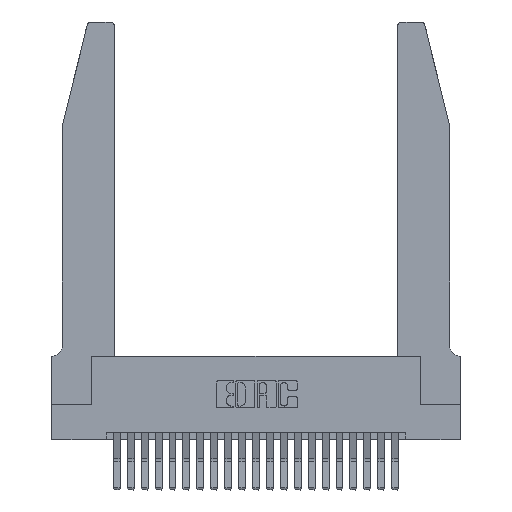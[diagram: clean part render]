
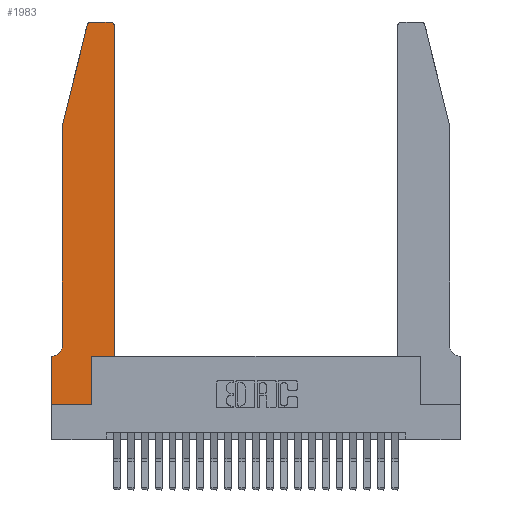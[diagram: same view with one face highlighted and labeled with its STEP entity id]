
A CAD part, top view. The second image highlights one B-rep face of the part: STEP entity #1983.
In plain terms, the highlighted planar face has unit normal (0, 0, 1).
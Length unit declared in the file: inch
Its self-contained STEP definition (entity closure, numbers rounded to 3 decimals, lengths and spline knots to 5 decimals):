
#393 = CARTESIAN_POINT ( 'NONE',  ( 0.25487, 2.72718, 0.37 ) ) ;
#771 = CARTESIAN_POINT ( 'NONE',  ( 0.4505, 0.35, 0.37 ) ) ;
#783 = VECTOR ( 'NONE', #19299, 39.37008 ) ;
#787 = CARTESIAN_POINT ( 'NONE',  ( 0.0755, 2., 0.37 ) ) ;
#1270 = EDGE_CURVE ( 'NONE', #22218, #2845, #3159, .T. ) ;
#1387 = LINE ( 'NONE', #17428, #783 ) ;
#1776 = CARTESIAN_POINT ( 'NONE',  ( 0.4505, 2.72, 0.37 ) ) ;
#1844 = EDGE_CURVE ( 'NONE', #18925, #15972, #16262, .T. ) ;
#1957 = EDGE_CURVE ( 'NONE', #10190, #18925, #10724, .T. ) ;
#1972 = DIRECTION ( 'NONE',  ( 0., 0., -1. ) ) ;
#1983 = ADVANCED_FACE ( 'NONE', ( #2831 ), #7440, .T. ) ;
#2825 = CARTESIAN_POINT ( 'NONE',  ( 0.0755, 2., 0.37 ) ) ;
#2831 = FACE_OUTER_BOUND ( 'NONE', #17076, .T. ) ;
#2845 = VERTEX_POINT ( 'NONE', #771 ) ;
#3020 = ORIENTED_EDGE ( 'NONE', *, *, #17323, .T. ) ;
#3159 = LINE ( 'NONE', #14717, #12492 ) ;
#3385 = EDGE_CURVE ( 'NONE', #19134, #23123, #23197, .T. ) ;
#3589 = CARTESIAN_POINT ( 'NONE',  ( 0., 0., 0.37 ) ) ;
#3640 = CARTESIAN_POINT ( 'NONE',  ( 0.2865, 0., 0.37 ) ) ;
#4093 = LINE ( 'NONE', #12165, #12855 ) ;
#4153 = CARTESIAN_POINT ( 'NONE',  ( 0.0755, 0.42, 0.37 ) ) ;
#4448 = AXIS2_PLACEMENT_3D ( 'NONE', #9465, #22510, #11345 ) ;
#4659 = CIRCLE ( 'NONE', #4448, 0.03 ) ;
#4950 = CARTESIAN_POINT ( 'NONE',  ( 0.4205, 2.75, 0.37 ) ) ;
#5473 = DIRECTION ( 'NONE',  ( 0., -1., 0. ) ) ;
#5679 = ORIENTED_EDGE ( 'NONE', *, *, #6315, .T. ) ;
#6129 = VERTEX_POINT ( 'NONE', #1776 ) ;
#6315 = EDGE_CURVE ( 'NONE', #14402, #19134, #6682, .T. ) ;
#6682 = LINE ( 'NONE', #2825, #15990 ) ;
#7050 = CARTESIAN_POINT ( 'NONE',  ( 0., 0., 0.37 ) ) ;
#7345 = ORIENTED_EDGE ( 'NONE', *, *, #1957, .T. ) ;
#7440 = PLANE ( 'NONE',  #12505 ) ;
#7567 = CARTESIAN_POINT ( 'NONE',  ( 0., 0.35, 0.37 ) ) ;
#8650 = VECTOR ( 'NONE', #14544, 39.37008 ) ;
#8851 = CARTESIAN_POINT ( 'NONE',  ( 0.4505, 0.35, 0.37 ) ) ;
#9111 = CARTESIAN_POINT ( 'NONE',  ( 0.284, 2.75, 0.37 ) ) ;
#9291 = DIRECTION ( 'NONE',  ( 0., 0., 1. ) ) ;
#9465 = CARTESIAN_POINT ( 'NONE',  ( 0.4205, 2.72, 0.37 ) ) ;
#9630 = VECTOR ( 'NONE', #13015, 39.37008 ) ;
#9710 = AXIS2_PLACEMENT_3D ( 'NONE', #13144, #1972, #15028 ) ;
#9763 = ORIENTED_EDGE ( 'NONE', *, *, #18154, .T. ) ;
#9809 = LINE ( 'NONE', #8851, #8650 ) ;
#9981 = CARTESIAN_POINT ( 'NONE',  ( 0.284, 2.72, 0.37 ) ) ;
#10190 = VERTEX_POINT ( 'NONE', #7567 ) ;
#10262 = ORIENTED_EDGE ( 'NONE', *, *, #18262, .T. ) ;
#10686 = CIRCLE ( 'NONE', #9710, 0.07 ) ;
#10724 = LINE ( 'NONE', #3589, #13318 ) ;
#10831 = ORIENTED_EDGE ( 'NONE', *, *, #1844, .T. ) ;
#11131 = ORIENTED_EDGE ( 'NONE', *, *, #21164, .T. ) ;
#11345 = DIRECTION ( 'NONE',  ( 1., 0., 0. ) ) ;
#11694 = CARTESIAN_POINT ( 'NONE',  ( 0.0755, 2., 0.37 ) ) ;
#11853 = DIRECTION ( 'NONE',  ( 1., 0., 0. ) ) ;
#12165 = CARTESIAN_POINT ( 'NONE',  ( 0.0755, 0.35, 0.37 ) ) ;
#12492 = VECTOR ( 'NONE', #18353, 39.37008 ) ;
#12505 = AXIS2_PLACEMENT_3D ( 'NONE', #20451, #9291, #22352 ) ;
#12855 = VECTOR ( 'NONE', #23268, 39.37008 ) ;
#12883 = CARTESIAN_POINT ( 'NONE',  ( 0., 0., 0.37 ) ) ;
#13015 = DIRECTION ( 'NONE',  ( -1., 0., 0. ) ) ;
#13144 = CARTESIAN_POINT ( 'NONE',  ( 0.0055, 0.42, 0.37 ) ) ;
#13263 = VECTOR ( 'NONE', #13549, 39.37008 ) ;
#13318 = VECTOR ( 'NONE', #5473, 39.37008 ) ;
#13424 = CARTESIAN_POINT ( 'NONE',  ( 0.2865, 0.35, 0.37 ) ) ;
#13549 = DIRECTION ( 'NONE',  ( 0., -1., 0. ) ) ;
#13806 = VERTEX_POINT ( 'NONE', #19394 ) ;
#14402 = VERTEX_POINT ( 'NONE', #393 ) ;
#14544 = DIRECTION ( 'NONE',  ( 0., 1., 0. ) ) ;
#14717 = CARTESIAN_POINT ( 'NONE',  ( 0.4505, 0.35, 0.37 ) ) ;
#14800 = ORIENTED_EDGE ( 'NONE', *, *, #3385, .T. ) ;
#14899 = CARTESIAN_POINT ( 'NONE',  ( 0.2605, 2.75, 0.37 ) ) ;
#15028 = DIRECTION ( 'NONE',  ( -1., 0., 0. ) ) ;
#15187 = CIRCLE ( 'NONE', #20963, 0.03 ) ;
#15672 = VECTOR ( 'NONE', #20046, 39.37008 ) ;
#15874 = DIRECTION ( 'NONE',  ( -0.239, -0.971, 0. ) ) ;
#15972 = VERTEX_POINT ( 'NONE', #3640 ) ;
#15990 = VECTOR ( 'NONE', #15874, 39.37008 ) ;
#16262 = LINE ( 'NONE', #7050, #15672 ) ;
#17076 = EDGE_LOOP ( 'NONE', ( #20058, #11131, #5679, #14800, #10262, #18146, #7345, #10831, #3020, #22729, #9763, #18793 ) ) ;
#17323 = EDGE_CURVE ( 'NONE', #15972, #22218, #1387, .T. ) ;
#17428 = CARTESIAN_POINT ( 'NONE',  ( 0.2865, 0.35, 0.37 ) ) ;
#18146 = ORIENTED_EDGE ( 'NONE', *, *, #21317, .T. ) ;
#18154 = EDGE_CURVE ( 'NONE', #2845, #6129, #9809, .T. ) ;
#18262 = EDGE_CURVE ( 'NONE', #23123, #13806, #10686, .T. ) ;
#18353 = DIRECTION ( 'NONE',  ( 1., 0., 0. ) ) ;
#18793 = ORIENTED_EDGE ( 'NONE', *, *, #22941, .T. ) ;
#18925 = VERTEX_POINT ( 'NONE', #12883 ) ;
#19134 = VERTEX_POINT ( 'NONE', #787 ) ;
#19299 = DIRECTION ( 'NONE',  ( 0., 1., 0. ) ) ;
#19394 = CARTESIAN_POINT ( 'NONE',  ( 0.0055, 0.35, 0.37 ) ) ;
#19474 = VERTEX_POINT ( 'NONE', #9111 ) ;
#19521 = LINE ( 'NONE', #14899, #9630 ) ;
#20046 = DIRECTION ( 'NONE',  ( 1., 0., 0. ) ) ;
#20058 = ORIENTED_EDGE ( 'NONE', *, *, #23594, .T. ) ;
#20451 = CARTESIAN_POINT ( 'NONE',  ( 0., 0.35, 0.37 ) ) ;
#20963 = AXIS2_PLACEMENT_3D ( 'NONE', #9981, #23024, #11853 ) ;
#21164 = EDGE_CURVE ( 'NONE', #19474, #14402, #15187, .T. ) ;
#21317 = EDGE_CURVE ( 'NONE', #13806, #10190, #4093, .T. ) ;
#22218 = VERTEX_POINT ( 'NONE', #13424 ) ;
#22352 = DIRECTION ( 'NONE',  ( 1., 0., 0. ) ) ;
#22510 = DIRECTION ( 'NONE',  ( 0., 0., 1. ) ) ;
#22729 = ORIENTED_EDGE ( 'NONE', *, *, #1270, .T. ) ;
#22941 = EDGE_CURVE ( 'NONE', #6129, #23373, #4659, .T. ) ;
#23024 = DIRECTION ( 'NONE',  ( 0., 0., 1. ) ) ;
#23123 = VERTEX_POINT ( 'NONE', #4153 ) ;
#23197 = LINE ( 'NONE', #11694, #13263 ) ;
#23268 = DIRECTION ( 'NONE',  ( -1., 0., 0. ) ) ;
#23373 = VERTEX_POINT ( 'NONE', #4950 ) ;
#23594 = EDGE_CURVE ( 'NONE', #23373, #19474, #19521, .T. ) ;
